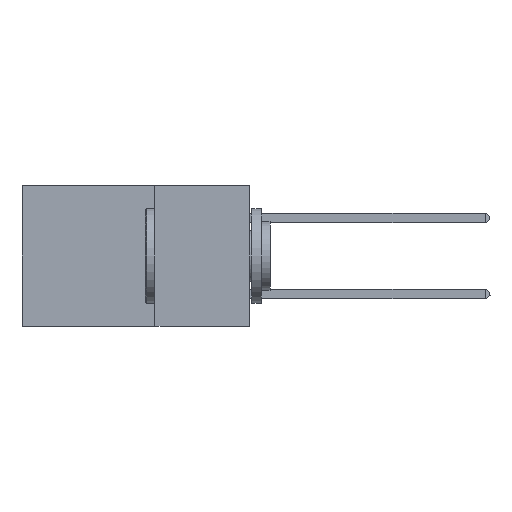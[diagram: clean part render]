
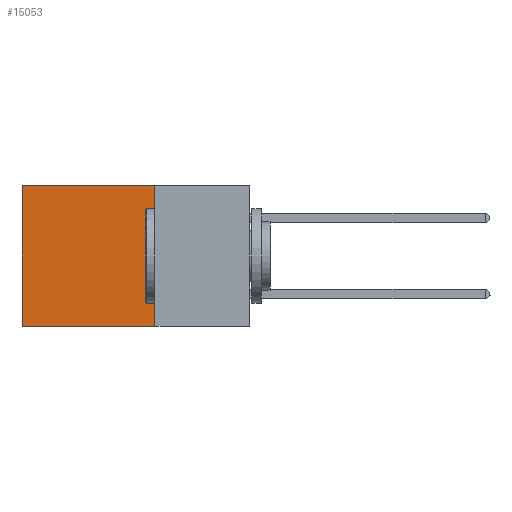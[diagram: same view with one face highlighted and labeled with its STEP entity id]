
A CAD part, left-side view. The second image highlights one B-rep face of the part: STEP entity #15053.
In plain terms, the highlighted planar face has unit normal (-1, 0, 0).
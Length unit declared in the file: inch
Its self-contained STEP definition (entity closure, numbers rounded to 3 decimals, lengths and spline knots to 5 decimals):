
#53 = VERTEX_POINT ( 'NONE', #16420 ) ;
#328 = VERTEX_POINT ( 'NONE', #13106 ) ;
#1314 = CARTESIAN_POINT ( 'NONE',  ( 0.2875, 0.6, 0. ) ) ;
#2622 = CARTESIAN_POINT ( 'NONE',  ( 0.2875, 0.25, 0. ) ) ;
#2726 = CARTESIAN_POINT ( 'NONE',  ( 0.2875, 0.25, 0. ) ) ;
#3494 = DIRECTION ( 'NONE',  ( 0., 0., -1. ) ) ;
#3793 = VECTOR ( 'NONE', #3494, 39.37008 ) ;
#3852 = LINE ( 'NONE', #1314, #18074 ) ;
#3907 = CARTESIAN_POINT ( 'NONE',  ( 0.2875, 0.25, 0. ) ) ;
#4024 = ORIENTED_EDGE ( 'NONE', *, *, #7794, .F. ) ;
#5919 = EDGE_CURVE ( 'NONE', #53, #328, #3852, .T. ) ;
#5923 = VECTOR ( 'NONE', #17613, 39.37008 ) ;
#6169 = LINE ( 'NONE', #3907, #6380 ) ;
#6380 = VECTOR ( 'NONE', #14645, 39.37008 ) ;
#6764 = CARTESIAN_POINT ( 'NONE',  ( 0.2875, 0.25, -0.37 ) ) ;
#7155 = PLANE ( 'NONE',  #15607 ) ;
#7353 = DIRECTION ( 'NONE',  ( 0., 0., -1. ) ) ;
#7422 = CARTESIAN_POINT ( 'NONE',  ( 0.2875, 0.25, -0.37 ) ) ;
#7471 = DIRECTION ( 'NONE',  ( 0., 0., -1. ) ) ;
#7794 = EDGE_CURVE ( 'NONE', #9937, #14171, #18035, .T. ) ;
#9937 = VERTEX_POINT ( 'NONE', #2726 ) ;
#10258 = DIRECTION ( 'NONE',  ( 1., 0., 0. ) ) ;
#11201 = ORIENTED_EDGE ( 'NONE', *, *, #5919, .T. ) ;
#12221 = EDGE_CURVE ( 'NONE', #14171, #328, #19923, .T. ) ;
#12503 = FACE_OUTER_BOUND ( 'NONE', #17426, .T. ) ;
#13106 = CARTESIAN_POINT ( 'NONE',  ( 0.2875, 0.6, -0.37 ) ) ;
#14171 = VERTEX_POINT ( 'NONE', #7422 ) ;
#14645 = DIRECTION ( 'NONE',  ( 0., 1., 0. ) ) ;
#15053 = ADVANCED_FACE ( 'NONE', ( #12503 ), #7155, .F. ) ;
#15607 = AXIS2_PLACEMENT_3D ( 'NONE', #2622, #10258, #7353 ) ;
#15631 = CARTESIAN_POINT ( 'NONE',  ( 0.2875, 0.25, 0. ) ) ;
#16409 = ORIENTED_EDGE ( 'NONE', *, *, #17512, .T. ) ;
#16420 = CARTESIAN_POINT ( 'NONE',  ( 0.2875, 0.6, 0. ) ) ;
#17426 = EDGE_LOOP ( 'NONE', ( #11201, #18900, #4024, #16409 ) ) ;
#17512 = EDGE_CURVE ( 'NONE', #9937, #53, #6169, .T. ) ;
#17613 = DIRECTION ( 'NONE',  ( 0., 1., 0. ) ) ;
#18035 = LINE ( 'NONE', #15631, #3793 ) ;
#18074 = VECTOR ( 'NONE', #7471, 39.37008 ) ;
#18900 = ORIENTED_EDGE ( 'NONE', *, *, #12221, .F. ) ;
#19923 = LINE ( 'NONE', #6764, #5923 ) ;
